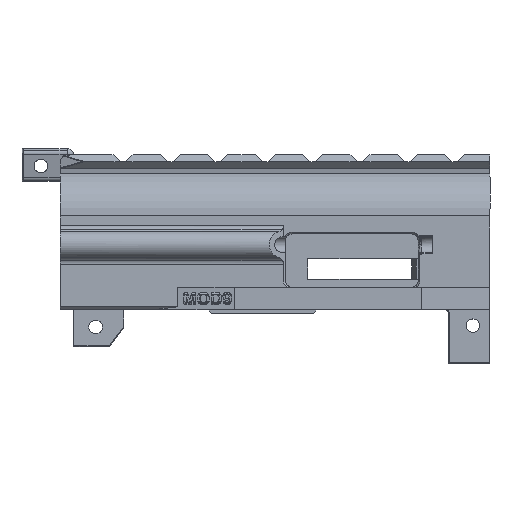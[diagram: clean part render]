
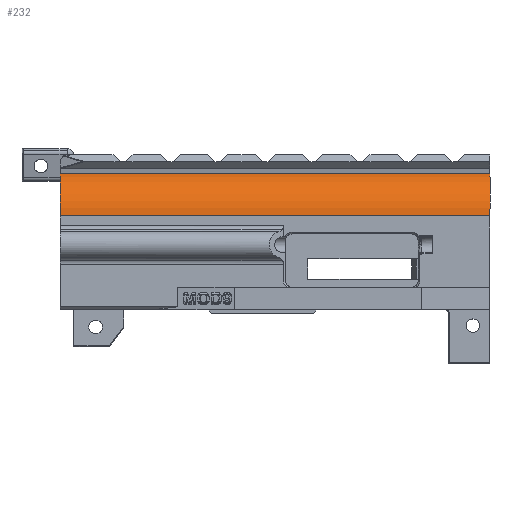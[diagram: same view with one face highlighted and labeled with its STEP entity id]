
A CAD part, top view. The second image highlights one B-rep face of the part: STEP entity #232.
In plain terms, the highlighted cylindrical face has radius 20.1 mm (diameter 40.2 mm), a partial arc.
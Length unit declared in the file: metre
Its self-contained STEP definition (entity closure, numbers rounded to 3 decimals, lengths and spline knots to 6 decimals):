
#232=ADVANCED_FACE('0:1231',(#983),#984,.T.);
#983=FACE_OUTER_BOUND('',#2126,.T.);
#984=CYLINDRICAL_SURFACE('',#2127,0.0201);
#2126=EDGE_LOOP('',(#5661,#5662,#5663,#5664));
#2127=AXIS2_PLACEMENT_3D('',#5665,#5666,#5667);
#5661=ORIENTED_EDGE('',*,*,#9319,.T.);
#5662=ORIENTED_EDGE('',*,*,#9093,.T.);
#5663=ORIENTED_EDGE('',*,*,#9318,.F.);
#5664=ORIENTED_EDGE('',*,*,#9200,.T.);
#5665=CARTESIAN_POINT('',(-0.020072,0.047361,0.001));
#5666=DIRECTION('',(-1.0,0.,0.));
#5667=DIRECTION('',(0.,0.,-1.0));
#9093=EDGE_CURVE('0:4870',#11176,#11174,#11177,.T.);
#9200=EDGE_CURVE('0:4876',#11357,#11355,#11358,.T.);
#9318=EDGE_CURVE('0:4873',#11357,#11174,#11536,.T.);
#9319=EDGE_CURVE('0:4864',#11355,#11176,#11537,.T.);
#11174=VERTEX_POINT('',#14681);
#11176=VERTEX_POINT('',#14684);
#11177=CIRCLE('',#14685,0.0201);
#11355=VERTEX_POINT('',#14948);
#11357=VERTEX_POINT('',#14951);
#11358=CIRCLE('',#14952,0.0201);
#11536=LINE('',#15252,#15253);
#11537=LINE('',#15254,#15255);
#14681=CARTESIAN_POINT('',(-0.178704,0.047361,0.0211));
#14684=CARTESIAN_POINT('',(-0.178704,0.065991,0.008545));
#14685=AXIS2_PLACEMENT_3D('',#19348,#19349,#19350);
#14948=CARTESIAN_POINT('',(0.011678,0.065991,0.008545));
#14951=CARTESIAN_POINT('',(0.011678,0.047361,0.0211));
#14952=AXIS2_PLACEMENT_3D('',#19497,#19498,#19499);
#15252=CARTESIAN_POINT('',(-0.020072,0.047361,0.0211));
#15253=VECTOR('',#19675,0.190382);
#15254=CARTESIAN_POINT('',(-0.020072,0.065991,0.008545));
#15255=VECTOR('',#19676,0.190382);
#19348=CARTESIAN_POINT('',(-0.178704,0.047361,0.001));
#19349=DIRECTION('',(1.0,0.,0.));
#19350=DIRECTION('',(0.,0.,-1.0));
#19497=CARTESIAN_POINT('',(0.011678,0.047361,0.001));
#19498=DIRECTION('',(-1.0,0.,0.));
#19499=DIRECTION('',(0.,0.,-1.0));
#19675=DIRECTION('',(-1.0,0.0,0.));
#19676=DIRECTION('',(-1.0,0.0,0.));
